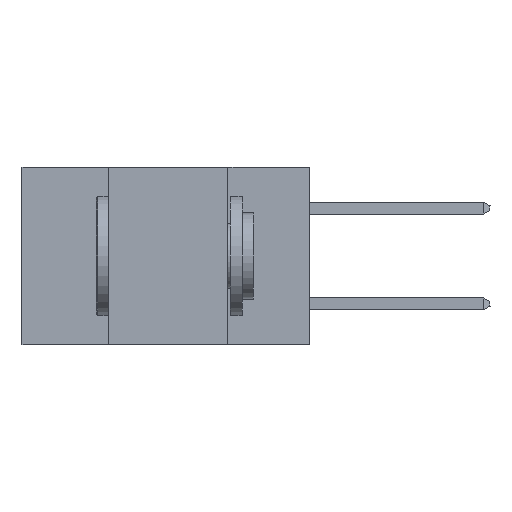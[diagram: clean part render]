
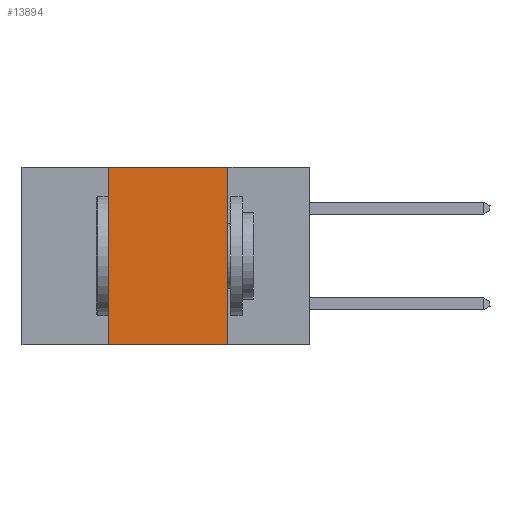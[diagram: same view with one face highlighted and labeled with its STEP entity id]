
A CAD part, left-side view. The second image highlights one B-rep face of the part: STEP entity #13894.
In plain terms, the highlighted planar face has unit normal (-1, 0, 0).
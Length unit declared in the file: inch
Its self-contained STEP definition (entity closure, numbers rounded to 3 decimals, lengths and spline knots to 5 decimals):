
#177 = CARTESIAN_POINT ( 'NONE',  ( 0., 0.6, 0. ) ) ;
#1073 = LINE ( 'NONE', #22556, #15704 ) ;
#3070 = DIRECTION ( 'NONE',  ( 1., 0., 0. ) ) ;
#4015 = CARTESIAN_POINT ( 'NONE',  ( 0., 0.6, 0. ) ) ;
#6573 = DIRECTION ( 'NONE',  ( 0., 0., -1. ) ) ;
#10383 = FACE_OUTER_BOUND ( 'NONE', #19666, .T. ) ;
#10410 = VECTOR ( 'NONE', #25500, 39.37008 ) ;
#10660 = CARTESIAN_POINT ( 'NONE',  ( 0., 0.17, -0.37 ) ) ;
#12150 = DIRECTION ( 'NONE',  ( 0., -1., 0. ) ) ;
#13175 = CARTESIAN_POINT ( 'NONE',  ( 0., 0.17, 0. ) ) ;
#13894 = ADVANCED_FACE ( 'NONE', ( #10383 ), #27886, .F. ) ;
#14011 = DIRECTION ( 'NONE',  ( 0., -1., 0. ) ) ;
#15704 = VECTOR ( 'NONE', #12150, 39.37008 ) ;
#15864 = VERTEX_POINT ( 'NONE', #10660 ) ;
#16471 = VERTEX_POINT ( 'NONE', #18272 ) ;
#16568 = VERTEX_POINT ( 'NONE', #18845 ) ;
#18272 = CARTESIAN_POINT ( 'NONE',  ( 0., 0.42, -0.37 ) ) ;
#18377 = AXIS2_PLACEMENT_3D ( 'NONE', #177, #3070, #6573 ) ;
#18845 = CARTESIAN_POINT ( 'NONE',  ( 0., 0.17, 0. ) ) ;
#19614 = EDGE_CURVE ( 'NONE', #16471, #15864, #1073, .T. ) ;
#19666 = EDGE_LOOP ( 'NONE', ( #23794, #32829, #20258, #27876 ) ) ;
#20258 = ORIENTED_EDGE ( 'NONE', *, *, #32695, .F. ) ;
#20992 = VECTOR ( 'NONE', #41137, 39.37008 ) ;
#21397 = CARTESIAN_POINT ( 'NONE',  ( 0., 0.42, 0. ) ) ;
#21440 = LINE ( 'NONE', #4015, #25239 ) ;
#22556 = CARTESIAN_POINT ( 'NONE',  ( 0., 0.6, -0.37 ) ) ;
#23794 = ORIENTED_EDGE ( 'NONE', *, *, #26888, .F. ) ;
#25239 = VECTOR ( 'NONE', #14011, 39.37008 ) ;
#25500 = DIRECTION ( 'NONE',  ( 0., 0., 1. ) ) ;
#26888 = EDGE_CURVE ( 'NONE', #16568, #15864, #26993, .T. ) ;
#26993 = LINE ( 'NONE', #13175, #20992 ) ;
#27757 = EDGE_CURVE ( 'NONE', #28602, #16568, #21440, .T. ) ;
#27876 = ORIENTED_EDGE ( 'NONE', *, *, #19614, .T. ) ;
#27886 = PLANE ( 'NONE',  #18377 ) ;
#28602 = VERTEX_POINT ( 'NONE', #33845 ) ;
#32695 = EDGE_CURVE ( 'NONE', #16471, #28602, #40664, .T. ) ;
#32829 = ORIENTED_EDGE ( 'NONE', *, *, #27757, .F. ) ;
#33845 = CARTESIAN_POINT ( 'NONE',  ( 0., 0.42, 0. ) ) ;
#40664 = LINE ( 'NONE', #21397, #10410 ) ;
#41137 = DIRECTION ( 'NONE',  ( 0., 0., -1. ) ) ;
